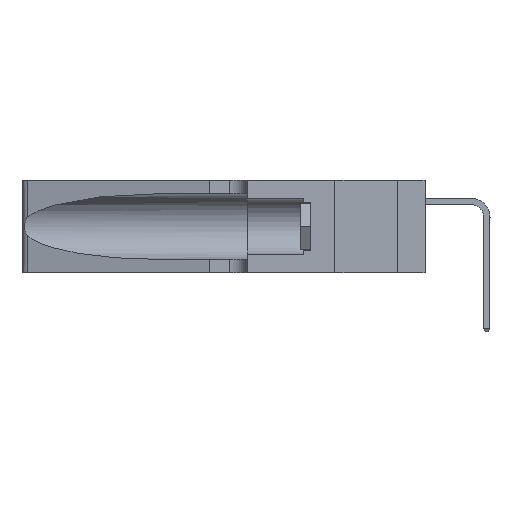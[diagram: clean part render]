
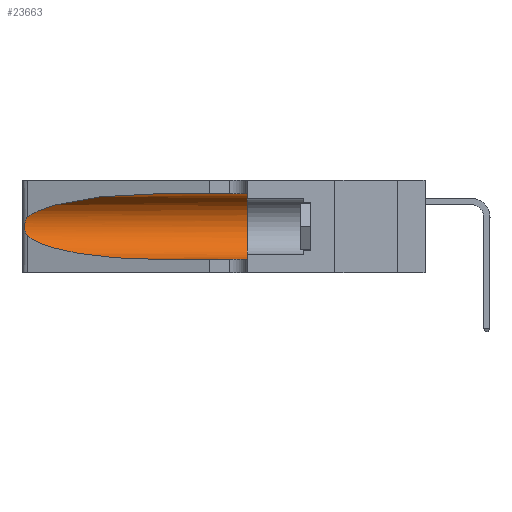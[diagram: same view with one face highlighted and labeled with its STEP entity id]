
A CAD part, left-side view. The second image highlights one B-rep face of the part: STEP entity #23663.
In plain terms, the highlighted cylindrical face has radius 3.308 mm (diameter 6.617 mm), a partial arc.
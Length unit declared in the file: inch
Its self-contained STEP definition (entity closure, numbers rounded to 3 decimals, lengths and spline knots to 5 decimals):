
#546 = EDGE_CURVE ( 'NONE', #25512, #15535, #28258, .T. ) ;
#579 = VECTOR ( 'NONE', #6451, 39.37008 ) ;
#885 = CARTESIAN_POINT ( 'NONE',  ( 0.25787, 1.23484, 0.2124 ) ) ;
#1168 = VERTEX_POINT ( 'NONE', #30307 ) ;
#1357 = ORIENTED_EDGE ( 'NONE', *, *, #9919, .T. ) ;
#1566 = VERTEX_POINT ( 'NONE', #27620 ) ;
#2806 = CARTESIAN_POINT ( 'NONE',  ( 0.1305, 0.35, 0.31525 ) ) ;
#3113 = VERTEX_POINT ( 'NONE', #39917 ) ;
#3188 = VERTEX_POINT ( 'NONE', #43718 ) ;
#3363 = B_SPLINE_CURVE_WITH_KNOTS ( 'NONE', 3,
 ( #39055, #42552, #21692, #885, #25134, #4412, #28627, #7919, #32141, #11403, #35669, #14898, #39212, #18387 ),
 .UNSPECIFIED., .F., .F.,
 ( 4, 2, 2, 2, 2, 2, 4 ),
 ( 0., 0.00027, 0.00053, 0.00107, 0.0016, 0.00187, 0.00214 ),
 .UNSPECIFIED. ) ;
#4239 = CYLINDRICAL_SURFACE ( 'NONE', #25824, 0.13025 ) ;
#4412 = CARTESIAN_POINT ( 'NONE',  ( 0.26018, 1.23835, 0.19895 ) ) ;
#4454 = EDGE_CURVE ( 'NONE', #25512, #1168, #35881, .T. ) ;
#5259 = EDGE_CURVE ( 'NONE', #3113, #3188, #9926, .T. ) ;
#6451 = DIRECTION ( 'NONE',  ( 0., -1., 0. ) ) ;
#7351 = ORIENTED_EDGE ( 'NONE', *, *, #4454, .T. ) ;
#7919 = CARTESIAN_POINT ( 'NONE',  ( 0.26075, 1.23896, 0.178 ) ) ;
#8176 = EDGE_CURVE ( 'NONE', #15535, #3188, #17763, .T. ) ;
#9271 = CARTESIAN_POINT ( 'NONE',  ( 0.1305, 0.35, 0.185 ) ) ;
#9647 = CARTESIAN_POINT ( 'NONE',  ( 0.1305, 1.61858, 0.31525 ) ) ;
#9919 = EDGE_CURVE ( 'NONE', #1168, #1566, #3363, .T. ) ;
#9926 = LINE ( 'NONE', #42186, #44722 ) ;
#10164 = ORIENTED_EDGE ( 'NONE', *, *, #37903, .T. ) ;
#11403 = CARTESIAN_POINT ( 'NONE',  ( 0.25856, 1.23593, 0.16098 ) ) ;
#11433 = CARTESIAN_POINT ( 'NONE',  ( 0.18966, 0.96281, 0.05475 ) ) ;
#12769 = DIRECTION ( 'NONE',  ( 0., 0., 1. ) ) ;
#13695 = CARTESIAN_POINT ( 'NONE',  ( 0.1305, 0.72297, 0.31525 ) ) ;
#14898 = CARTESIAN_POINT ( 'NONE',  ( 0.25639, 1.23186, 0.15144 ) ) ;
#15535 = VERTEX_POINT ( 'NONE', #2806 ) ;
#15647 =( BOUNDED_CURVE ( )  B_SPLINE_CURVE ( 3, ( #42574, #28653, #11433, #35699 ),
 .UNSPECIFIED., .F., .F. ) 
 B_SPLINE_CURVE_WITH_KNOTS ( ( 4, 4 ),
 ( 3.44316, 4.71239 ),
 .UNSPECIFIED. ) 
 CURVE ( )  GEOMETRIC_REPRESENTATION_ITEM ( )  RATIONAL_B_SPLINE_CURVE ( ( 1., 0.87, 0.87, 1. ) ) 
 REPRESENTATION_ITEM ( '' )  );
#15859 = EDGE_LOOP ( 'NONE', ( #7351, #1357, #10164, #25320, #41186, #34067 ) ) ;
#17181 = CARTESIAN_POINT ( 'NONE',  ( 0.2373, 1.15595, 0.28018 ) ) ;
#17763 = CIRCLE ( 'NONE', #20052, 0.13025 ) ;
#18387 = CARTESIAN_POINT ( 'NONE',  ( 0.25487, 1.22718, 0.14631 ) ) ;
#20052 = AXIS2_PLACEMENT_3D ( 'NONE', #9271, #33513, #12769 ) ;
#20723 = DIRECTION ( 'NONE',  ( 0., 0., -1. ) ) ;
#21692 = CARTESIAN_POINT ( 'NONE',  ( 0.25639, 1.23184, 0.21858 ) ) ;
#23663 = ADVANCED_FACE ( 'NONE', ( #41193 ), #4239, .F. ) ;
#25134 = CARTESIAN_POINT ( 'NONE',  ( 0.25854, 1.2359, 0.20912 ) ) ;
#25320 = ORIENTED_EDGE ( 'NONE', *, *, #5259, .T. ) ;
#25512 = VERTEX_POINT ( 'NONE', #31139 ) ;
#25824 = AXIS2_PLACEMENT_3D ( 'NONE', #38052, #45083, #20723 ) ;
#27620 = CARTESIAN_POINT ( 'NONE',  ( 0.25487, 1.22718, 0.14631 ) ) ;
#28258 = LINE ( 'NONE', #9647, #579 ) ;
#28627 = CARTESIAN_POINT ( 'NONE',  ( 0.26075, 1.23896, 0.19203 ) ) ;
#28653 = CARTESIAN_POINT ( 'NONE',  ( 0.2373, 1.15595, 0.08982 ) ) ;
#30307 = CARTESIAN_POINT ( 'NONE',  ( 0.25487, 1.22718, 0.22369 ) ) ;
#31139 = CARTESIAN_POINT ( 'NONE',  ( 0.1305, 0.72297, 0.31525 ) ) ;
#32141 = CARTESIAN_POINT ( 'NONE',  ( 0.26017, 1.23833, 0.17102 ) ) ;
#33513 = DIRECTION ( 'NONE',  ( 0., 1., 0. ) ) ;
#34067 = ORIENTED_EDGE ( 'NONE', *, *, #546, .F. ) ;
#35150 = DIRECTION ( 'NONE',  ( 0., -1., 0. ) ) ;
#35669 = CARTESIAN_POINT ( 'NONE',  ( 0.25789, 1.23486, 0.15765 ) ) ;
#35699 = CARTESIAN_POINT ( 'NONE',  ( 0.1305, 0.72297, 0.05475 ) ) ;
#35881 =( BOUNDED_CURVE ( )  B_SPLINE_CURVE ( 3, ( #13695, #37980, #17181, #41483 ),
 .UNSPECIFIED., .F., .F. ) 
 B_SPLINE_CURVE_WITH_KNOTS ( ( 4, 4 ),
 ( 1.5708, 2.84003 ),
 .UNSPECIFIED. ) 
 CURVE ( )  GEOMETRIC_REPRESENTATION_ITEM ( )  RATIONAL_B_SPLINE_CURVE ( ( 1., 0.87, 0.87, 1. ) ) 
 REPRESENTATION_ITEM ( '' )  );
#37903 = EDGE_CURVE ( 'NONE', #1566, #3113, #15647, .T. ) ;
#37980 = CARTESIAN_POINT ( 'NONE',  ( 0.18966, 0.96281, 0.31525 ) ) ;
#38052 = CARTESIAN_POINT ( 'NONE',  ( 0.1305, 1.61858, 0.185 ) ) ;
#39055 = CARTESIAN_POINT ( 'NONE',  ( 0.25487, 1.22718, 0.22369 ) ) ;
#39212 = CARTESIAN_POINT ( 'NONE',  ( 0.25555, 1.22993, 0.14849 ) ) ;
#39917 = CARTESIAN_POINT ( 'NONE',  ( 0.1305, 0.72297, 0.05475 ) ) ;
#41186 = ORIENTED_EDGE ( 'NONE', *, *, #8176, .F. ) ;
#41193 = FACE_OUTER_BOUND ( 'NONE', #15859, .T. ) ;
#41483 = CARTESIAN_POINT ( 'NONE',  ( 0.25487, 1.22718, 0.22369 ) ) ;
#42186 = CARTESIAN_POINT ( 'NONE',  ( 0.1305, 1.61858, 0.05475 ) ) ;
#42552 = CARTESIAN_POINT ( 'NONE',  ( 0.25555, 1.22994, 0.2215 ) ) ;
#42574 = CARTESIAN_POINT ( 'NONE',  ( 0.25487, 1.22718, 0.14631 ) ) ;
#43718 = CARTESIAN_POINT ( 'NONE',  ( 0.1305, 0.35, 0.05475 ) ) ;
#44722 = VECTOR ( 'NONE', #35150, 39.37008 ) ;
#45083 = DIRECTION ( 'NONE',  ( 0., -1., 0. ) ) ;
